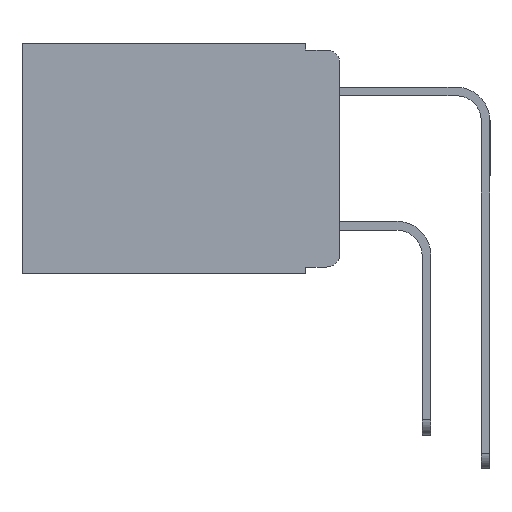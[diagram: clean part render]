
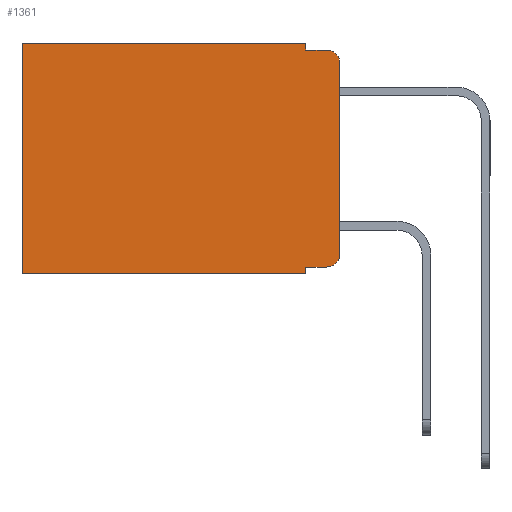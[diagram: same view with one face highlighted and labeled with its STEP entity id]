
A CAD part, left-side view. The second image highlights one B-rep face of the part: STEP entity #1361.
In plain terms, the highlighted planar face has unit normal (-1, 0, 0).
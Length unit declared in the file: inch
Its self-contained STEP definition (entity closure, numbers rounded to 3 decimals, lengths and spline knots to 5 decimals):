
#31 = EDGE_CURVE ( 'NONE', #6137, #18641, #16052, .T. ) ;
#111 = FACE_OUTER_BOUND ( 'NONE', #6475, .T. ) ;
#271 = DIRECTION ( 'NONE',  ( 0., 0., -1. ) ) ;
#732 = CARTESIAN_POINT ( 'NONE',  ( 0.298, 0.051, 0. ) ) ;
#735 = LINE ( 'NONE', #4409, #4742 ) ;
#1019 = VERTEX_POINT ( 'NONE', #16105 ) ;
#1121 = VECTOR ( 'NONE', #14744, 39.37008 ) ;
#1361 = ADVANCED_FACE ( 'NONE', ( #111 ), #16332, .F. ) ;
#1966 = CARTESIAN_POINT ( 'NONE',  ( 0.298, 0., 0. ) ) ;
#2076 = DIRECTION ( 'NONE',  ( -1., 0., 0. ) ) ;
#2101 = LINE ( 'NONE', #6604, #14760 ) ;
#2502 = DIRECTION ( 'NONE',  ( 0., 0., -1. ) ) ;
#2673 = CARTESIAN_POINT ( 'NONE',  ( 0.298, 0.473, 0. ) ) ;
#3360 = CARTESIAN_POINT ( 'NONE',  ( 0.298, 0.051, -0.01 ) ) ;
#3390 = ORIENTED_EDGE ( 'NONE', *, *, #4120, .T. ) ;
#3633 = CARTESIAN_POINT ( 'NONE',  ( 0.298, 0., -0.03 ) ) ;
#3639 = AXIS2_PLACEMENT_3D ( 'NONE', #16435, #18939, #7410 ) ;
#3899 = DIRECTION ( 'NONE',  ( 0., 0., -1. ) ) ;
#4120 = EDGE_CURVE ( 'NONE', #5218, #1019, #6621, .T. ) ;
#4409 = CARTESIAN_POINT ( 'NONE',  ( 0.298, 0.051, -0.333 ) ) ;
#4715 = CARTESIAN_POINT ( 'NONE',  ( 0.298, 0.051, -0.01 ) ) ;
#4742 = VECTOR ( 'NONE', #11071, 39.37008 ) ;
#5218 = VERTEX_POINT ( 'NONE', #9228 ) ;
#6137 = VERTEX_POINT ( 'NONE', #3633 ) ;
#6169 = EDGE_CURVE ( 'NONE', #11165, #18641, #8466, .T. ) ;
#6368 = DIRECTION ( 'NONE',  ( 0., -1., 0. ) ) ;
#6475 = EDGE_LOOP ( 'NONE', ( #7716, #18868, #19366, #6717, #3390, #18429, #20407, #17968, #18446, #11444 ) ) ;
#6604 = CARTESIAN_POINT ( 'NONE',  ( 0.298, 0.051, 0. ) ) ;
#6621 = LINE ( 'NONE', #18346, #14839 ) ;
#6638 = CARTESIAN_POINT ( 'NONE',  ( 0.298, 0.02, -0.01 ) ) ;
#6717 = ORIENTED_EDGE ( 'NONE', *, *, #14984, .F. ) ;
#7007 = DIRECTION ( 'NONE',  ( 0., 1., 0. ) ) ;
#7369 = CARTESIAN_POINT ( 'NONE',  ( 0.298, 0.02, -0.333 ) ) ;
#7410 = DIRECTION ( 'NONE',  ( 0., 0., -1. ) ) ;
#7640 = LINE ( 'NONE', #4715, #15342 ) ;
#7716 = ORIENTED_EDGE ( 'NONE', *, *, #31, .F. ) ;
#8068 = VECTOR ( 'NONE', #2502, 39.37008 ) ;
#8122 = AXIS2_PLACEMENT_3D ( 'NONE', #12029, #2076, #13653 ) ;
#8378 = EDGE_CURVE ( 'NONE', #17207, #11165, #735, .T. ) ;
#8466 = CIRCLE ( 'NONE', #8122, 0.02 ) ;
#9228 = CARTESIAN_POINT ( 'NONE',  ( 0.298, 0.051, 0. ) ) ;
#9525 = EDGE_CURVE ( 'NONE', #17207, #16572, #2101, .T. ) ;
#9800 = CARTESIAN_POINT ( 'NONE',  ( 0.298, 0.051, -0.343 ) ) ;
#9941 = DIRECTION ( 'NONE',  ( 0., 0., -1. ) ) ;
#10023 = CARTESIAN_POINT ( 'NONE',  ( 0.298, 0., -0.313 ) ) ;
#10357 = DIRECTION ( 'NONE',  ( -1., 0., 0. ) ) ;
#10624 = EDGE_CURVE ( 'NONE', #1019, #17276, #15160, .T. ) ;
#11071 = DIRECTION ( 'NONE',  ( 0., -1., 0. ) ) ;
#11165 = VERTEX_POINT ( 'NONE', #7369 ) ;
#11198 = CIRCLE ( 'NONE', #19912, 0.02 ) ;
#11444 = ORIENTED_EDGE ( 'NONE', *, *, #6169, .T. ) ;
#11747 = VECTOR ( 'NONE', #3899, 39.37008 ) ;
#12013 = EDGE_CURVE ( 'NONE', #16572, #17276, #18576, .T. ) ;
#12029 = CARTESIAN_POINT ( 'NONE',  ( 0.298, 0.02, -0.313 ) ) ;
#12592 = DIRECTION ( 'NONE',  ( 0., 0., -1. ) ) ;
#13653 = DIRECTION ( 'NONE',  ( 0., 0., -1. ) ) ;
#14162 = VECTOR ( 'NONE', #12592, 39.37008 ) ;
#14744 = DIRECTION ( 'NONE',  ( 0., 1., 0. ) ) ;
#14760 = VECTOR ( 'NONE', #9941, 39.37008 ) ;
#14839 = VECTOR ( 'NONE', #7007, 39.37008 ) ;
#14984 = EDGE_CURVE ( 'NONE', #5218, #15917, #16737, .T. ) ;
#15160 = LINE ( 'NONE', #2673, #14162 ) ;
#15342 = VECTOR ( 'NONE', #6368, 39.37008 ) ;
#15917 = VERTEX_POINT ( 'NONE', #3360 ) ;
#16052 = LINE ( 'NONE', #1966, #11747 ) ;
#16105 = CARTESIAN_POINT ( 'NONE',  ( 0.298, 0.473, 0. ) ) ;
#16332 = PLANE ( 'NONE',  #3639 ) ;
#16343 = CARTESIAN_POINT ( 'NONE',  ( 0.298, 0., -0.343 ) ) ;
#16435 = CARTESIAN_POINT ( 'NONE',  ( 0.298, 0., 0. ) ) ;
#16572 = VERTEX_POINT ( 'NONE', #9800 ) ;
#16580 = CARTESIAN_POINT ( 'NONE',  ( 0.298, 0.473, -0.343 ) ) ;
#16737 = LINE ( 'NONE', #732, #8068 ) ;
#17093 = EDGE_CURVE ( 'NONE', #15917, #19824, #7640, .T. ) ;
#17207 = VERTEX_POINT ( 'NONE', #19605 ) ;
#17276 = VERTEX_POINT ( 'NONE', #16580 ) ;
#17968 = ORIENTED_EDGE ( 'NONE', *, *, #9525, .F. ) ;
#18346 = CARTESIAN_POINT ( 'NONE',  ( 0.298, 0., 0. ) ) ;
#18429 = ORIENTED_EDGE ( 'NONE', *, *, #10624, .T. ) ;
#18446 = ORIENTED_EDGE ( 'NONE', *, *, #8378, .T. ) ;
#18576 = LINE ( 'NONE', #16343, #1121 ) ;
#18641 = VERTEX_POINT ( 'NONE', #10023 ) ;
#18868 = ORIENTED_EDGE ( 'NONE', *, *, #19213, .T. ) ;
#18939 = DIRECTION ( 'NONE',  ( 1., 0., 0. ) ) ;
#19213 = EDGE_CURVE ( 'NONE', #6137, #19824, #11198, .T. ) ;
#19366 = ORIENTED_EDGE ( 'NONE', *, *, #17093, .F. ) ;
#19605 = CARTESIAN_POINT ( 'NONE',  ( 0.298, 0.051, -0.333 ) ) ;
#19824 = VERTEX_POINT ( 'NONE', #6638 ) ;
#19912 = AXIS2_PLACEMENT_3D ( 'NONE', #19925, #10357, #271 ) ;
#19925 = CARTESIAN_POINT ( 'NONE',  ( 0.298, 0.02, -0.03 ) ) ;
#20407 = ORIENTED_EDGE ( 'NONE', *, *, #12013, .F. ) ;
